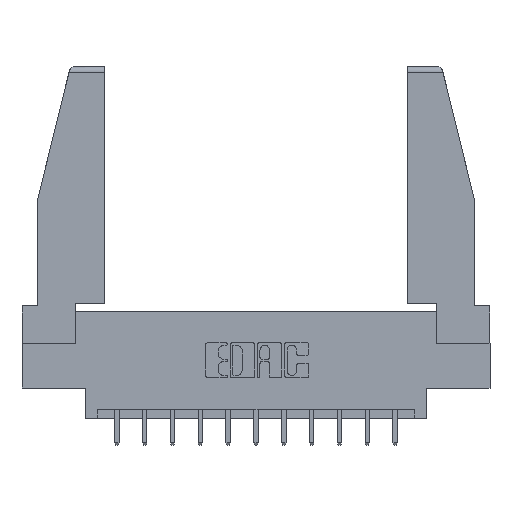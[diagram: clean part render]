
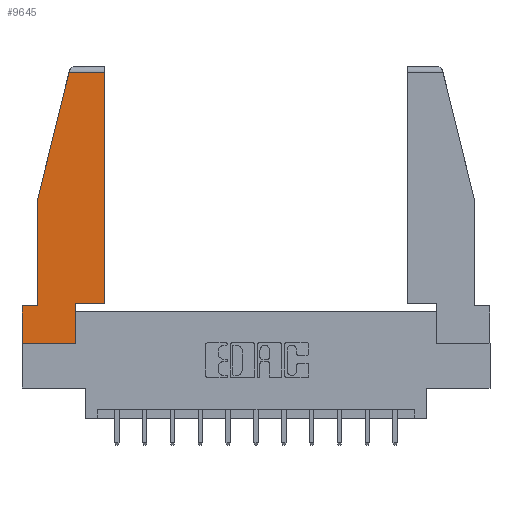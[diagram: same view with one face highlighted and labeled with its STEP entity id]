
A CAD part, top view. The second image highlights one B-rep face of the part: STEP entity #9645.
In plain terms, the highlighted planar face has unit normal (0, 0, 1).
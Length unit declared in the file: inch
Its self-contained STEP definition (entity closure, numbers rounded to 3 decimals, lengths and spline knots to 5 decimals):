
#148 = CARTESIAN_POINT ( 'NONE',  ( 0.461, 0.223, 0. ) ) ;
#258 = LINE ( 'NONE', #10938, #3350 ) ;
#422 = EDGE_CURVE ( 'NONE', #3050, #2576, #6168, .T. ) ;
#528 = LINE ( 'NONE', #4258, #12941 ) ;
#576 = PLANE ( 'NONE',  #2968 ) ;
#747 = EDGE_CURVE ( 'NONE', #8468, #15044, #842, .T. ) ;
#842 = LINE ( 'NONE', #2898, #4321 ) ;
#972 = CARTESIAN_POINT ( 'NONE',  ( 0., 0., 0. ) ) ;
#982 = CARTESIAN_POINT ( 'NONE',  ( 0.086, 0.21, 0. ) ) ;
#1099 = FACE_OUTER_BOUND ( 'NONE', #7125, .T. ) ;
#1343 = LINE ( 'NONE', #12393, #2619 ) ;
#2249 = EDGE_CURVE ( 'NONE', #2576, #6475, #258, .T. ) ;
#2489 = CARTESIAN_POINT ( 'NONE',  ( 0.297, 0.223, 0. ) ) ;
#2576 = VERTEX_POINT ( 'NONE', #972 ) ;
#2619 = VECTOR ( 'NONE', #3173, 39.37008 ) ;
#2862 = VECTOR ( 'NONE', #5863, 39.37008 ) ;
#2898 = CARTESIAN_POINT ( 'NONE',  ( 0., 1.52, 0. ) ) ;
#2925 = DIRECTION ( 'NONE',  ( 1., 0., 0. ) ) ;
#2968 = AXIS2_PLACEMENT_3D ( 'NONE', #9773, #9883, #2925 ) ;
#3050 = VERTEX_POINT ( 'NONE', #11810 ) ;
#3173 = DIRECTION ( 'NONE',  ( -1., 0., 0. ) ) ;
#3308 = DIRECTION ( 'NONE',  ( -0.239, -0.971, 0. ) ) ;
#3350 = VECTOR ( 'NONE', #9540, 39.37008 ) ;
#3825 = ORIENTED_EDGE ( 'NONE', *, *, #5596, .T. ) ;
#3956 = VERTEX_POINT ( 'NONE', #9177 ) ;
#4082 = DIRECTION ( 'NONE',  ( -1., 0., 0. ) ) ;
#4258 = CARTESIAN_POINT ( 'NONE',  ( 0.297, 0., 0. ) ) ;
#4321 = VECTOR ( 'NONE', #4082, 39.37008 ) ;
#4347 = ORIENTED_EDGE ( 'NONE', *, *, #4655, .T. ) ;
#4655 = EDGE_CURVE ( 'NONE', #7426, #8468, #7407, .T. ) ;
#5119 = VERTEX_POINT ( 'NONE', #2489 ) ;
#5596 = EDGE_CURVE ( 'NONE', #12786, #3050, #1343, .T. ) ;
#5863 = DIRECTION ( 'NONE',  ( 0., -1., 0. ) ) ;
#6168 = LINE ( 'NONE', #8975, #2862 ) ;
#6475 = VERTEX_POINT ( 'NONE', #8649 ) ;
#7125 = EDGE_LOOP ( 'NONE', ( #4347, #13507, #8366, #7431, #3825, #7801, #14912, #7503, #7677 ) ) ;
#7245 = CARTESIAN_POINT ( 'NONE',  ( 0.2636, 1.52, 0. ) ) ;
#7407 = LINE ( 'NONE', #8976, #12509 ) ;
#7426 = VERTEX_POINT ( 'NONE', #148 ) ;
#7431 = ORIENTED_EDGE ( 'NONE', *, *, #14744, .T. ) ;
#7503 = ORIENTED_EDGE ( 'NONE', *, *, #13296, .T. ) ;
#7677 = ORIENTED_EDGE ( 'NONE', *, *, #12883, .T. ) ;
#7780 = CARTESIAN_POINT ( 'NONE',  ( 0.086, 0.8, 0. ) ) ;
#7801 = ORIENTED_EDGE ( 'NONE', *, *, #422, .T. ) ;
#8228 = VECTOR ( 'NONE', #3308, 39.37008 ) ;
#8366 = ORIENTED_EDGE ( 'NONE', *, *, #14236, .T. ) ;
#8468 = VERTEX_POINT ( 'NONE', #11293 ) ;
#8595 = LINE ( 'NONE', #7780, #12044 ) ;
#8649 = CARTESIAN_POINT ( 'NONE',  ( 0.297, 0., 0. ) ) ;
#8938 = DIRECTION ( 'NONE',  ( 0., 1., 0. ) ) ;
#8975 = CARTESIAN_POINT ( 'NONE',  ( 0., 0.21, 0. ) ) ;
#8976 = CARTESIAN_POINT ( 'NONE',  ( 0.461, 0.223, 0. ) ) ;
#8985 = LINE ( 'NONE', #13982, #14071 ) ;
#9177 = CARTESIAN_POINT ( 'NONE',  ( 0.086, 0.8, 0. ) ) ;
#9540 = DIRECTION ( 'NONE',  ( 1., 0., 0. ) ) ;
#9645 = ADVANCED_FACE ( 'NONE', ( #1099 ), #576, .T. ) ;
#9773 = CARTESIAN_POINT ( 'NONE',  ( 0., 0., 0. ) ) ;
#9883 = DIRECTION ( 'NONE',  ( 0., 0., 1. ) ) ;
#10280 = CARTESIAN_POINT ( 'NONE',  ( 0.271, 1.55, 0. ) ) ;
#10457 = DIRECTION ( 'NONE',  ( 1., 0., 0. ) ) ;
#10938 = CARTESIAN_POINT ( 'NONE',  ( 0., 0., 0. ) ) ;
#10975 = LINE ( 'NONE', #10280, #8228 ) ;
#11293 = CARTESIAN_POINT ( 'NONE',  ( 0.461, 1.52, 0. ) ) ;
#11810 = CARTESIAN_POINT ( 'NONE',  ( 0., 0.21, 0. ) ) ;
#12044 = VECTOR ( 'NONE', #12421, 39.37008 ) ;
#12393 = CARTESIAN_POINT ( 'NONE',  ( 0., 0.21, 0. ) ) ;
#12421 = DIRECTION ( 'NONE',  ( 0., -1., 0. ) ) ;
#12509 = VECTOR ( 'NONE', #13653, 39.37008 ) ;
#12786 = VERTEX_POINT ( 'NONE', #982 ) ;
#12883 = EDGE_CURVE ( 'NONE', #5119, #7426, #8985, .T. ) ;
#12941 = VECTOR ( 'NONE', #8938, 39.37008 ) ;
#13296 = EDGE_CURVE ( 'NONE', #6475, #5119, #528, .T. ) ;
#13507 = ORIENTED_EDGE ( 'NONE', *, *, #747, .T. ) ;
#13653 = DIRECTION ( 'NONE',  ( 0., 1., 0. ) ) ;
#13982 = CARTESIAN_POINT ( 'NONE',  ( 0.297, 0.223, 0. ) ) ;
#14071 = VECTOR ( 'NONE', #10457, 39.37008 ) ;
#14236 = EDGE_CURVE ( 'NONE', #15044, #3956, #10975, .T. ) ;
#14744 = EDGE_CURVE ( 'NONE', #3956, #12786, #8595, .T. ) ;
#14912 = ORIENTED_EDGE ( 'NONE', *, *, #2249, .T. ) ;
#15044 = VERTEX_POINT ( 'NONE', #7245 ) ;
